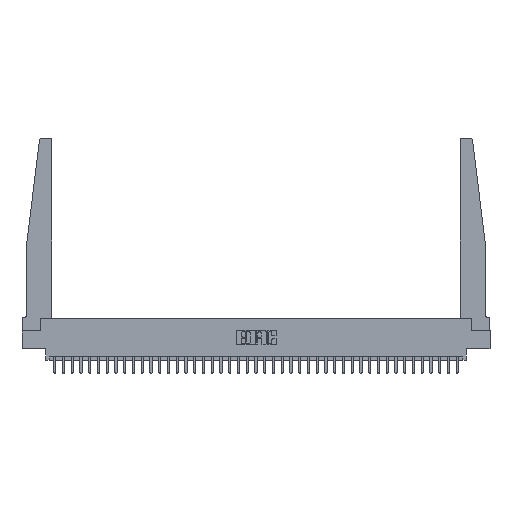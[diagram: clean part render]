
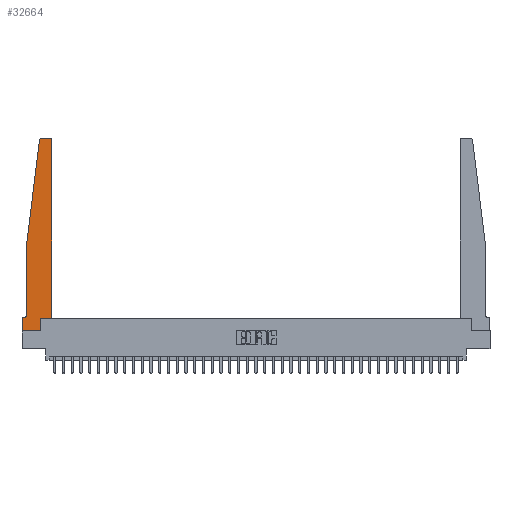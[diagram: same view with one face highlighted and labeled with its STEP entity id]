
A CAD part, top view. The second image highlights one B-rep face of the part: STEP entity #32664.
In plain terms, the highlighted planar face has unit normal (0, 0, 1).
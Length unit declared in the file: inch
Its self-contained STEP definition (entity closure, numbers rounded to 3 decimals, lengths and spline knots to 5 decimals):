
#543 = DIRECTION ( 'NONE',  ( 0., -1., 0. ) ) ;
#623 = CARTESIAN_POINT ( 'NONE',  ( 0., 0., 0.37 ) ) ;
#828 = ORIENTED_EDGE ( 'NONE', *, *, #10419, .T. ) ;
#982 = EDGE_LOOP ( 'NONE', ( #22877, #10401, #25707, #828, #31791, #10349, #16492, #9439, #28554, #2727, #33775, #5081 ) ) ;
#1065 = CARTESIAN_POINT ( 'NONE',  ( 0.395, 2.75, 0.37 ) ) ;
#1251 = LINE ( 'NONE', #17106, #5389 ) ;
#1361 = VERTEX_POINT ( 'NONE', #3924 ) ;
#1507 = DIRECTION ( 'NONE',  ( -1., 0., 0. ) ) ;
#2173 = CARTESIAN_POINT ( 'NONE',  ( 0.015, 0.1875, 0.37 ) ) ;
#2582 = VERTEX_POINT ( 'NONE', #623 ) ;
#2727 = ORIENTED_EDGE ( 'NONE', *, *, #27254, .T. ) ;
#2900 = VECTOR ( 'NONE', #1507, 39.37008 ) ;
#3015 = CARTESIAN_POINT ( 'NONE',  ( 0.27653, 2.75, 0.37 ) ) ;
#3363 = VECTOR ( 'NONE', #23353, 39.37008 ) ;
#3597 = VERTEX_POINT ( 'NONE', #16698 ) ;
#3706 = CARTESIAN_POINT ( 'NONE',  ( 0., 0.1875, 0.37 ) ) ;
#3924 = CARTESIAN_POINT ( 'NONE',  ( 0.065, 1.25, 0.37 ) ) ;
#3982 = DIRECTION ( 'NONE',  ( -1., 0., 0. ) ) ;
#4013 = VECTOR ( 'NONE', #3982, 39.37008 ) ;
#4163 = CARTESIAN_POINT ( 'NONE',  ( 0., 0., 0.37 ) ) ;
#4226 = VERTEX_POINT ( 'NONE', #3706 ) ;
#5081 = ORIENTED_EDGE ( 'NONE', *, *, #25019, .T. ) ;
#5370 = VERTEX_POINT ( 'NONE', #3015 ) ;
#5389 = VECTOR ( 'NONE', #543, 39.37008 ) ;
#5453 = DIRECTION ( 'NONE',  ( 1., 0., 0. ) ) ;
#5664 = CARTESIAN_POINT ( 'NONE',  ( 0.2605, 0., 0.37 ) ) ;
#6030 = CARTESIAN_POINT ( 'NONE',  ( 0.425, 2.72, 0.37 ) ) ;
#6111 = AXIS2_PLACEMENT_3D ( 'NONE', #20613, #15429, #26172 ) ;
#6394 = EDGE_CURVE ( 'NONE', #2582, #11534, #12581, .T. ) ;
#6493 = CARTESIAN_POINT ( 'NONE',  ( 0.065, 1.25, 0.37 ) ) ;
#6738 = VERTEX_POINT ( 'NONE', #33828 ) ;
#6852 = EDGE_CURVE ( 'NONE', #5370, #33008, #10283, .T. ) ;
#7824 = CARTESIAN_POINT ( 'NONE',  ( 0.24675, 2.72367, 0.37 ) ) ;
#8077 = LINE ( 'NONE', #13283, #29615 ) ;
#8315 = EDGE_CURVE ( 'NONE', #21298, #5370, #18230, .T. ) ;
#8732 = VERTEX_POINT ( 'NONE', #2173 ) ;
#9372 = CARTESIAN_POINT ( 'NONE',  ( 0.065, 0.2375, 0.37 ) ) ;
#9439 = ORIENTED_EDGE ( 'NONE', *, *, #6394, .T. ) ;
#9722 = DIRECTION ( 'NONE',  ( 0., 1., 0. ) ) ;
#10283 = CIRCLE ( 'NONE', #34904, 0.03 ) ;
#10349 = ORIENTED_EDGE ( 'NONE', *, *, #35071, .T. ) ;
#10401 = ORIENTED_EDGE ( 'NONE', *, *, #6852, .T. ) ;
#10419 = EDGE_CURVE ( 'NONE', #1361, #21240, #31053, .T. ) ;
#10847 = CIRCLE ( 'NONE', #20582, 0.03 ) ;
#11331 = DIRECTION ( 'NONE',  ( -0.122, -0.992, 0. ) ) ;
#11534 = VERTEX_POINT ( 'NONE', #5664 ) ;
#12169 = DIRECTION ( 'NONE',  ( 1., 0., 0. ) ) ;
#12581 = LINE ( 'NONE', #4163, #3363 ) ;
#13049 = VECTOR ( 'NONE', #9722, 39.37008 ) ;
#13283 = CARTESIAN_POINT ( 'NONE',  ( 0.2605, 0.18, 0.37 ) ) ;
#13820 = DIRECTION ( 'NONE',  ( 0., 1., 0. ) ) ;
#14146 = CARTESIAN_POINT ( 'NONE',  ( 0., 0.1875, 0.37 ) ) ;
#14296 = DIRECTION ( 'NONE',  ( 0., 0., 1. ) ) ;
#14475 = CARTESIAN_POINT ( 'NONE',  ( 0.27653, 2.72, 0.37 ) ) ;
#15429 = DIRECTION ( 'NONE',  ( 0., 0., -1. ) ) ;
#16097 = VECTOR ( 'NONE', #17454, 39.37008 ) ;
#16492 = ORIENTED_EDGE ( 'NONE', *, *, #32421, .T. ) ;
#16698 = CARTESIAN_POINT ( 'NONE',  ( 0.2605, 0.18, 0.37 ) ) ;
#17106 = CARTESIAN_POINT ( 'NONE',  ( 0., 0., 0.37 ) ) ;
#17454 = DIRECTION ( 'NONE',  ( 0., -1., 0. ) ) ;
#17984 = VERTEX_POINT ( 'NONE', #6030 ) ;
#18230 = LINE ( 'NONE', #29318, #2900 ) ;
#18688 = LINE ( 'NONE', #20835, #13049 ) ;
#18975 = VECTOR ( 'NONE', #12169, 39.37008 ) ;
#19232 = EDGE_CURVE ( 'NONE', #21240, #8732, #32442, .T. ) ;
#19702 = DIRECTION ( 'NONE',  ( 0., 0., 1. ) ) ;
#20259 = EDGE_CURVE ( 'NONE', #11534, #3597, #8077, .T. ) ;
#20582 = AXIS2_PLACEMENT_3D ( 'NONE', #32905, #29830, #5453 ) ;
#20613 = CARTESIAN_POINT ( 'NONE',  ( 0.015, 0.2375, 0.37 ) ) ;
#20835 = CARTESIAN_POINT ( 'NONE',  ( 0.425, 0.18, 0.37 ) ) ;
#21240 = VERTEX_POINT ( 'NONE', #9372 ) ;
#21298 = VERTEX_POINT ( 'NONE', #1065 ) ;
#21931 = LINE ( 'NONE', #24971, #32714 ) ;
#22037 = PLANE ( 'NONE',  #27144 ) ;
#22877 = ORIENTED_EDGE ( 'NONE', *, *, #8315, .T. ) ;
#22916 = EDGE_CURVE ( 'NONE', #6738, #17984, #18688, .T. ) ;
#23353 = DIRECTION ( 'NONE',  ( 1., 0., 0. ) ) ;
#23357 = CARTESIAN_POINT ( 'NONE',  ( 0.065, 0.1875, 0.37 ) ) ;
#24971 = CARTESIAN_POINT ( 'NONE',  ( 0.065, 1.25, 0.37 ) ) ;
#25019 = EDGE_CURVE ( 'NONE', #17984, #21298, #10847, .T. ) ;
#25217 = DIRECTION ( 'NONE',  ( 1., 0., 0. ) ) ;
#25450 = CARTESIAN_POINT ( 'NONE',  ( 0.425, 0.18, 0.37 ) ) ;
#25698 = LINE ( 'NONE', #23357, #4013 ) ;
#25707 = ORIENTED_EDGE ( 'NONE', *, *, #26783, .T. ) ;
#26172 = DIRECTION ( 'NONE',  ( -1., 0., 0. ) ) ;
#26783 = EDGE_CURVE ( 'NONE', #33008, #1361, #21931, .T. ) ;
#27144 = AXIS2_PLACEMENT_3D ( 'NONE', #14146, #19702, #27571 ) ;
#27254 = EDGE_CURVE ( 'NONE', #3597, #6738, #34059, .T. ) ;
#27571 = DIRECTION ( 'NONE',  ( 1., 0., 0. ) ) ;
#28554 = ORIENTED_EDGE ( 'NONE', *, *, #20259, .T. ) ;
#29318 = CARTESIAN_POINT ( 'NONE',  ( 0.25, 2.75, 0.37 ) ) ;
#29615 = VECTOR ( 'NONE', #13820, 39.37008 ) ;
#29830 = DIRECTION ( 'NONE',  ( 0., 0., 1. ) ) ;
#30799 = FACE_OUTER_BOUND ( 'NONE', #982, .T. ) ;
#31053 = LINE ( 'NONE', #6493, #16097 ) ;
#31791 = ORIENTED_EDGE ( 'NONE', *, *, #19232, .T. ) ;
#32421 = EDGE_CURVE ( 'NONE', #4226, #2582, #1251, .T. ) ;
#32442 = CIRCLE ( 'NONE', #6111, 0.05 ) ;
#32664 = ADVANCED_FACE ( 'NONE', ( #30799 ), #22037, .T. ) ;
#32714 = VECTOR ( 'NONE', #11331, 39.37008 ) ;
#32905 = CARTESIAN_POINT ( 'NONE',  ( 0.395, 2.72, 0.37 ) ) ;
#33008 = VERTEX_POINT ( 'NONE', #7824 ) ;
#33775 = ORIENTED_EDGE ( 'NONE', *, *, #22916, .T. ) ;
#33828 = CARTESIAN_POINT ( 'NONE',  ( 0.425, 0.18, 0.37 ) ) ;
#34059 = LINE ( 'NONE', #25450, #18975 ) ;
#34904 = AXIS2_PLACEMENT_3D ( 'NONE', #14475, #14296, #25217 ) ;
#35071 = EDGE_CURVE ( 'NONE', #8732, #4226, #25698, .T. ) ;
